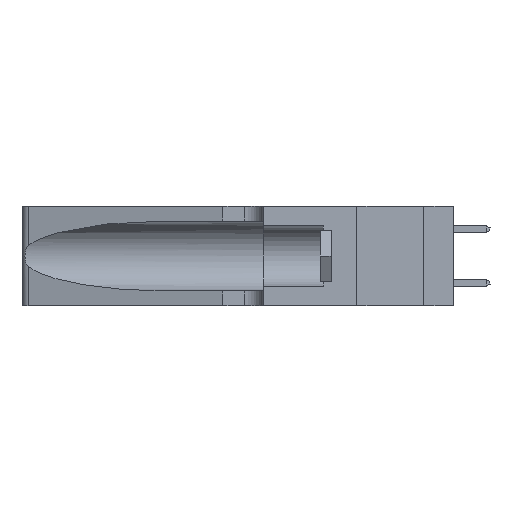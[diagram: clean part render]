
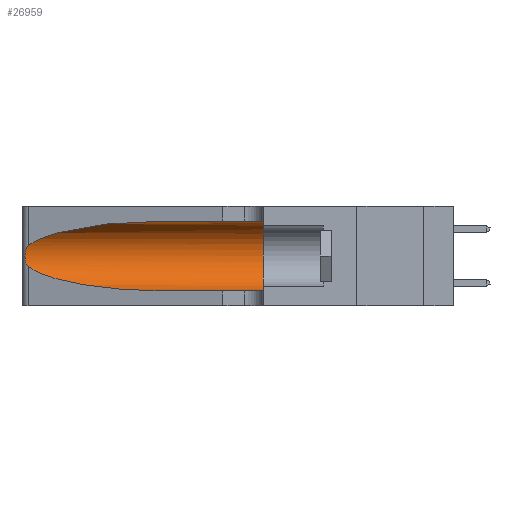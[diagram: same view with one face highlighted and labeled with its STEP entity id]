
A CAD part, left-side view. The second image highlights one B-rep face of the part: STEP entity #26959.
In plain terms, the highlighted cylindrical face has radius 3.308 mm (diameter 6.617 mm), a partial arc.
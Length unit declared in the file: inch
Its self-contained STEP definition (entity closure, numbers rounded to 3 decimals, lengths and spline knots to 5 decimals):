
#547 = CARTESIAN_POINT ( 'NONE',  ( 0.25487, 1.22718, 0.14631 ) ) ;
#881 = CARTESIAN_POINT ( 'NONE',  ( 0.1305, 0.72297, 0.31525 ) ) ;
#1380 = EDGE_CURVE ( 'NONE', #27905, #31939, #22358, .T. ) ;
#1653 = VERTEX_POINT ( 'NONE', #2272 ) ;
#2272 = CARTESIAN_POINT ( 'NONE',  ( 0.25487, 1.22718, 0.22369 ) ) ;
#2825 = CARTESIAN_POINT ( 'NONE',  ( 0.18966, 0.96281, 0.05475 ) ) ;
#2884 = FACE_OUTER_BOUND ( 'NONE', #12055, .T. ) ;
#3132 = ORIENTED_EDGE ( 'NONE', *, *, #22816, .T. ) ;
#3318 = CARTESIAN_POINT ( 'NONE',  ( 0.25639, 1.23184, 0.21858 ) ) ;
#6199 = CARTESIAN_POINT ( 'NONE',  ( 0.25854, 1.2359, 0.20912 ) ) ;
#6612 = DIRECTION ( 'NONE',  ( 0., -1., 0. ) ) ;
#7812 = EDGE_CURVE ( 'NONE', #30043, #25169, #18306, .T. ) ;
#8487 = CARTESIAN_POINT ( 'NONE',  ( 0.1305, 0.72297, 0.31525 ) ) ;
#8976 = CARTESIAN_POINT ( 'NONE',  ( 0.25555, 1.22994, 0.2215 ) ) ;
#9113 = CARTESIAN_POINT ( 'NONE',  ( 0.26075, 1.23896, 0.19203 ) ) ;
#9682 = ORIENTED_EDGE ( 'NONE', *, *, #7812, .T. ) ;
#11373 = CARTESIAN_POINT ( 'NONE',  ( 0.25487, 1.22718, 0.14631 ) ) ;
#11411 = CARTESIAN_POINT ( 'NONE',  ( 0.1305, 0.35, 0.185 ) ) ;
#11999 = CARTESIAN_POINT ( 'NONE',  ( 0.26017, 1.23833, 0.17102 ) ) ;
#12055 = EDGE_LOOP ( 'NONE', ( #3132, #30629, #17231, #9682, #26014, #28632 ) ) ;
#13402 = DIRECTION ( 'NONE',  ( 0., -1., 0. ) ) ;
#13530 = CARTESIAN_POINT ( 'NONE',  ( 0.1305, 1.61858, 0.185 ) ) ;
#14225 = B_SPLINE_CURVE_WITH_KNOTS ( 'NONE', 3,
 ( #14795, #8976, #3318, #23470, #6199, #26346, #9113, #29216, #11999, #32103, #14923, #35019, #17830, #547 ),
 .UNSPECIFIED., .F., .F.,
 ( 4, 2, 2, 2, 2, 2, 4 ),
 ( 0., 0.00027, 0.00053, 0.00107, 0.0016, 0.00187, 0.00214 ),
 .UNSPECIFIED. ) ;
#14293 = CARTESIAN_POINT ( 'NONE',  ( 0.2373, 1.15595, 0.08982 ) ) ;
#14311 = CARTESIAN_POINT ( 'NONE',  ( 0.2373, 1.15595, 0.28018 ) ) ;
#14329 = DIRECTION ( 'NONE',  ( 0., 0., 1. ) ) ;
#14720 = VECTOR ( 'NONE', #18459, 39.37008 ) ;
#14795 = CARTESIAN_POINT ( 'NONE',  ( 0.25487, 1.22718, 0.22369 ) ) ;
#14923 = CARTESIAN_POINT ( 'NONE',  ( 0.25789, 1.23486, 0.15765 ) ) ;
#15539 = CARTESIAN_POINT ( 'NONE',  ( 0.1305, 1.61858, 0.31525 ) ) ;
#17231 = ORIENTED_EDGE ( 'NONE', *, *, #27153, .T. ) ;
#17830 = CARTESIAN_POINT ( 'NONE',  ( 0.25555, 1.22993, 0.14849 ) ) ;
#18156 = CARTESIAN_POINT ( 'NONE',  ( 0.25487, 1.22718, 0.14631 ) ) ;
#18251 = CARTESIAN_POINT ( 'NONE',  ( 0.1305, 1.61858, 0.05475 ) ) ;
#18306 = LINE ( 'NONE', #18251, #32659 ) ;
#18459 = DIRECTION ( 'NONE',  ( 0., -1., 0. ) ) ;
#18741 = VERTEX_POINT ( 'NONE', #18156 ) ;
#18742 = CARTESIAN_POINT ( 'NONE',  ( 0.1305, 0.35, 0.05475 ) ) ;
#20935 =( BOUNDED_CURVE ( )  B_SPLINE_CURVE ( 3, ( #11373, #14293, #2825, #22972 ),
 .UNSPECIFIED., .F., .T. ) 
 B_SPLINE_CURVE_WITH_KNOTS ( ( 4, 4 ),
 ( 3.44316, 4.71239 ),
 .UNSPECIFIED. ) 
 CURVE ( )  GEOMETRIC_REPRESENTATION_ITEM ( )  RATIONAL_B_SPLINE_CURVE ( ( 1., 0.87, 0.87, 1. ) ) 
 REPRESENTATION_ITEM ( '' )  );
#21155 = CARTESIAN_POINT ( 'NONE',  ( 0.1305, 0.35, 0.31525 ) ) ;
#21693 = CARTESIAN_POINT ( 'NONE',  ( 0.1305, 0.72297, 0.05475 ) ) ;
#22358 = LINE ( 'NONE', #15539, #14720 ) ;
#22816 = EDGE_CURVE ( 'NONE', #27905, #1653, #34257, .T. ) ;
#22972 = CARTESIAN_POINT ( 'NONE',  ( 0.1305, 0.72297, 0.05475 ) ) ;
#23470 = CARTESIAN_POINT ( 'NONE',  ( 0.25787, 1.23484, 0.2124 ) ) ;
#24060 = CYLINDRICAL_SURFACE ( 'NONE', #30687, 0.13025 ) ;
#25169 = VERTEX_POINT ( 'NONE', #18742 ) ;
#26014 = ORIENTED_EDGE ( 'NONE', *, *, #29072, .F. ) ;
#26346 = CARTESIAN_POINT ( 'NONE',  ( 0.26018, 1.23835, 0.19895 ) ) ;
#26959 = ADVANCED_FACE ( 'NONE', ( #2884 ), #24060, .F. ) ;
#27153 = EDGE_CURVE ( 'NONE', #18741, #30043, #20935, .T. ) ;
#27284 = EDGE_CURVE ( 'NONE', #1653, #18741, #14225, .T. ) ;
#27905 = VERTEX_POINT ( 'NONE', #881 ) ;
#28632 = ORIENTED_EDGE ( 'NONE', *, *, #1380, .F. ) ;
#29072 = EDGE_CURVE ( 'NONE', #31939, #25169, #36891, .T. ) ;
#29216 = CARTESIAN_POINT ( 'NONE',  ( 0.26075, 1.23896, 0.178 ) ) ;
#30043 = VERTEX_POINT ( 'NONE', #21693 ) ;
#30629 = ORIENTED_EDGE ( 'NONE', *, *, #27284, .T. ) ;
#30687 = AXIS2_PLACEMENT_3D ( 'NONE', #13530, #13402, #36516 ) ;
#31516 = DIRECTION ( 'NONE',  ( 0., 1., 0. ) ) ;
#31939 = VERTEX_POINT ( 'NONE', #21155 ) ;
#32103 = CARTESIAN_POINT ( 'NONE',  ( 0.25856, 1.23593, 0.16098 ) ) ;
#32181 = AXIS2_PLACEMENT_3D ( 'NONE', #11411, #31516, #14329 ) ;
#32659 = VECTOR ( 'NONE', #6612, 39.37008 ) ;
#34257 =( BOUNDED_CURVE ( )  B_SPLINE_CURVE ( 3, ( #8487, #37149, #14311, #34416 ),
 .UNSPECIFIED., .F., .T. ) 
 B_SPLINE_CURVE_WITH_KNOTS ( ( 4, 4 ),
 ( 1.5708, 2.84003 ),
 .UNSPECIFIED. ) 
 CURVE ( )  GEOMETRIC_REPRESENTATION_ITEM ( )  RATIONAL_B_SPLINE_CURVE ( ( 1., 0.87, 0.87, 1. ) ) 
 REPRESENTATION_ITEM ( '' )  );
#34416 = CARTESIAN_POINT ( 'NONE',  ( 0.25487, 1.22718, 0.22369 ) ) ;
#35019 = CARTESIAN_POINT ( 'NONE',  ( 0.25639, 1.23186, 0.15144 ) ) ;
#36516 = DIRECTION ( 'NONE',  ( 0., 0., -1. ) ) ;
#36891 = CIRCLE ( 'NONE', #32181, 0.13025 ) ;
#37149 = CARTESIAN_POINT ( 'NONE',  ( 0.18966, 0.96281, 0.31525 ) ) ;
